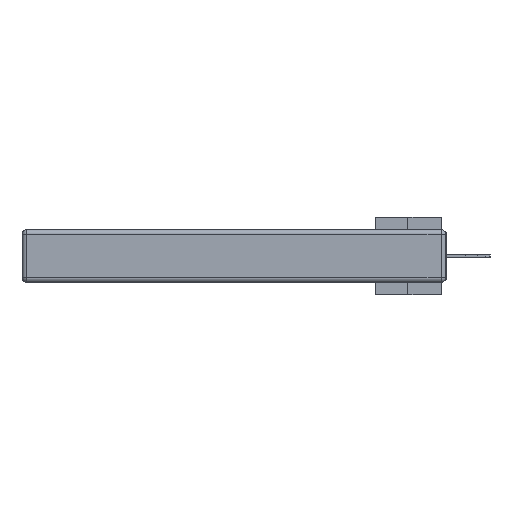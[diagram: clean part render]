
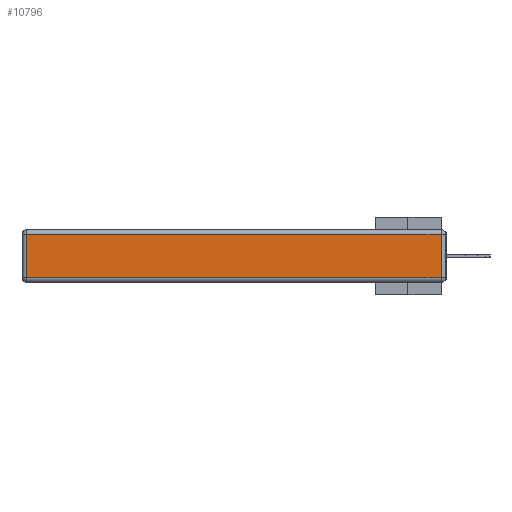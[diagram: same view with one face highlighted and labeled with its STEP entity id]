
A CAD part, left-side view. The second image highlights one B-rep face of the part: STEP entity #10796.
In plain terms, the highlighted planar face has unit normal (-1, 0, 0).
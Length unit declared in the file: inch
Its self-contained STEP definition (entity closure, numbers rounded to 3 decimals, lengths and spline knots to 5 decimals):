
#396 = CARTESIAN_POINT ( 'NONE',  ( 0., 0., -0.343 ) ) ;
#579 = PLANE ( 'NONE',  #12257 ) ;
#2291 = DIRECTION ( 'NONE',  ( 0., 1., 0. ) ) ;
#3680 = VERTEX_POINT ( 'NONE', #3727 ) ;
#3727 = CARTESIAN_POINT ( 'NONE',  ( 0., 2.72, -0.313 ) ) ;
#8002 = VECTOR ( 'NONE', #9364, 39.37008 ) ;
#8285 = VERTEX_POINT ( 'NONE', #24398 ) ;
#9326 = EDGE_CURVE ( 'NONE', #16508, #3680, #35922, .T. ) ;
#9364 = DIRECTION ( 'NONE',  ( 0., -1., 0. ) ) ;
#9639 = FACE_OUTER_BOUND ( 'NONE', #33518, .T. ) ;
#9677 = VECTOR ( 'NONE', #16150, 39.37008 ) ;
#9771 = LINE ( 'NONE', #33475, #9677 ) ;
#10796 = ADVANCED_FACE ( 'NONE', ( #9639 ), #579, .T. ) ;
#11624 = EDGE_CURVE ( 'NONE', #3680, #34266, #20758, .T. ) ;
#12058 = DIRECTION ( 'NONE',  ( 0., 0., -1. ) ) ;
#12257 = AXIS2_PLACEMENT_3D ( 'NONE', #396, #36023, #21614 ) ;
#13382 = CARTESIAN_POINT ( 'NONE',  ( 0., 0.03, -0.313 ) ) ;
#16150 = DIRECTION ( 'NONE',  ( 0., 0., 1. ) ) ;
#16508 = VERTEX_POINT ( 'NONE', #19790 ) ;
#19790 = CARTESIAN_POINT ( 'NONE',  ( 0., 2.72, -0.03 ) ) ;
#20440 = CARTESIAN_POINT ( 'NONE',  ( 0., 2.75, -0.03 ) ) ;
#20758 = LINE ( 'NONE', #26904, #8002 ) ;
#21614 = DIRECTION ( 'NONE',  ( 0., 0., 1. ) ) ;
#22005 = ORIENTED_EDGE ( 'NONE', *, *, #30853, .T. ) ;
#23314 = EDGE_CURVE ( 'NONE', #8285, #16508, #26028, .T. ) ;
#24398 = CARTESIAN_POINT ( 'NONE',  ( 0., 0.03, -0.03 ) ) ;
#24762 = ORIENTED_EDGE ( 'NONE', *, *, #9326, .T. ) ;
#26028 = LINE ( 'NONE', #20440, #28941 ) ;
#26904 = CARTESIAN_POINT ( 'NONE',  ( 0., 0., -0.313 ) ) ;
#28941 = VECTOR ( 'NONE', #2291, 39.37008 ) ;
#30409 = ORIENTED_EDGE ( 'NONE', *, *, #23314, .T. ) ;
#30853 = EDGE_CURVE ( 'NONE', #34266, #8285, #9771, .T. ) ;
#31481 = VECTOR ( 'NONE', #12058, 39.37008 ) ;
#31736 = ORIENTED_EDGE ( 'NONE', *, *, #11624, .T. ) ;
#32676 = CARTESIAN_POINT ( 'NONE',  ( 0., 2.72, -0.343 ) ) ;
#33475 = CARTESIAN_POINT ( 'NONE',  ( 0., 0.03, -0.343 ) ) ;
#33518 = EDGE_LOOP ( 'NONE', ( #31736, #22005, #30409, #24762 ) ) ;
#34266 = VERTEX_POINT ( 'NONE', #13382 ) ;
#35922 = LINE ( 'NONE', #32676, #31481 ) ;
#36023 = DIRECTION ( 'NONE',  ( -1., 0., 0. ) ) ;
